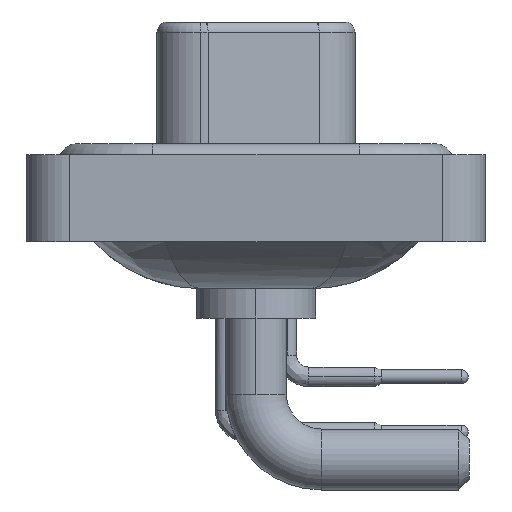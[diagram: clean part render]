
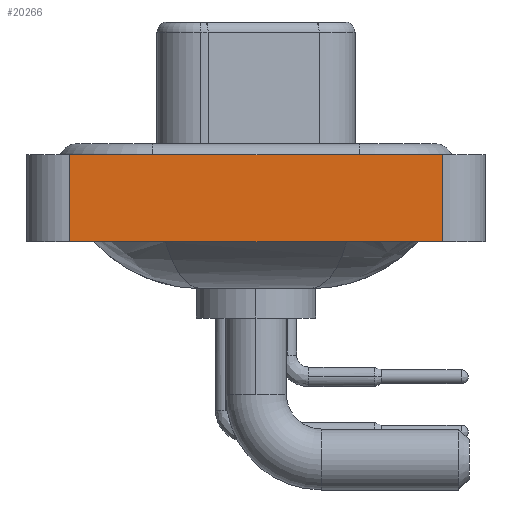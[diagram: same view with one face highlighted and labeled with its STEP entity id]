
A CAD part, left-side view. The second image highlights one B-rep face of the part: STEP entity #20266.
In plain terms, the highlighted planar face has unit normal (-1, 0, 0).
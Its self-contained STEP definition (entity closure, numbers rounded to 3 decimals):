
#761 = CARTESIAN_POINT ( 'NONE',  ( -7.35, 8.55, -3.6 ) ) ;
#1242 = LINE ( 'NONE', #23206, #27149 ) ;
#1544 = LINE ( 'NONE', #23924, #4000 ) ;
#1624 = EDGE_CURVE ( 'NONE', #17448, #13038, #1544, .T. ) ;
#1638 = AXIS2_PLACEMENT_3D ( 'NONE', #7548, #16275, #25050 ) ;
#2234 = CARTESIAN_POINT ( 'NONE',  ( -7.35, 8.55, -3.6 ) ) ;
#3544 = DIRECTION ( 'NONE',  ( 0., 0., 1. ) ) ;
#3686 = CARTESIAN_POINT ( 'NONE',  ( -7.35, 8.55, 0.4 ) ) ;
#4000 = VECTOR ( 'NONE', #18890, 1000. ) ;
#7223 = ORIENTED_EDGE ( 'NONE', *, *, #18401, .T. ) ;
#7548 = CARTESIAN_POINT ( 'NONE',  ( -7.35, -8.55, -3.6 ) ) ;
#7990 = CARTESIAN_POINT ( 'NONE',  ( -7.35, -8.55, 0.4 ) ) ;
#10772 = EDGE_CURVE ( 'NONE', #24080, #17448, #24860, .T. ) ;
#10892 = CARTESIAN_POINT ( 'NONE',  ( -7.35, -8.55, -3.6 ) ) ;
#11025 = EDGE_LOOP ( 'NONE', ( #25945, #13913, #23439, #7223 ) ) ;
#12226 = DIRECTION ( 'NONE',  ( 0., 0., 1. ) ) ;
#13038 = VERTEX_POINT ( 'NONE', #7990 ) ;
#13913 = ORIENTED_EDGE ( 'NONE', *, *, #1624, .F. ) ;
#14015 = VERTEX_POINT ( 'NONE', #23817 ) ;
#14808 = VECTOR ( 'NONE', #24507, 1000. ) ;
#15739 = LINE ( 'NONE', #10892, #14808 ) ;
#16275 = DIRECTION ( 'NONE',  ( -1., 0., 0. ) ) ;
#17433 = EDGE_CURVE ( 'NONE', #14015, #13038, #1242, .T. ) ;
#17448 = VERTEX_POINT ( 'NONE', #3686 ) ;
#18401 = EDGE_CURVE ( 'NONE', #24080, #14015, #15739, .T. ) ;
#18570 = FACE_OUTER_BOUND ( 'NONE', #11025, .T. ) ;
#18890 = DIRECTION ( 'NONE',  ( 0., -1., 0. ) ) ;
#20266 = ADVANCED_FACE ( 'NONE', ( #18570 ), #24628, .T. ) ;
#23206 = CARTESIAN_POINT ( 'NONE',  ( -7.35, -8.55, -3.6 ) ) ;
#23439 = ORIENTED_EDGE ( 'NONE', *, *, #10772, .F. ) ;
#23817 = CARTESIAN_POINT ( 'NONE',  ( -7.35, -8.55, -3.6 ) ) ;
#23924 = CARTESIAN_POINT ( 'NONE',  ( -7.35, -8.55, 0.4 ) ) ;
#24080 = VERTEX_POINT ( 'NONE', #2234 ) ;
#24507 = DIRECTION ( 'NONE',  ( 0., -1., 0. ) ) ;
#24628 = PLANE ( 'NONE',  #1638 ) ;
#24860 = LINE ( 'NONE', #761, #27724 ) ;
#25050 = DIRECTION ( 'NONE',  ( 0., 0., 1. ) ) ;
#25945 = ORIENTED_EDGE ( 'NONE', *, *, #17433, .T. ) ;
#27149 = VECTOR ( 'NONE', #3544, 1000. ) ;
#27724 = VECTOR ( 'NONE', #12226, 1000. ) ;
